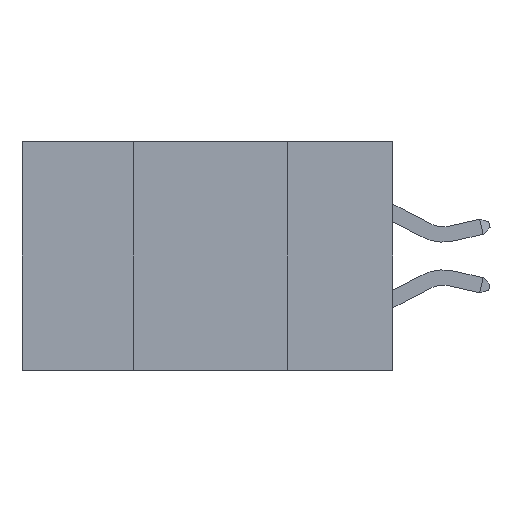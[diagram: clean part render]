
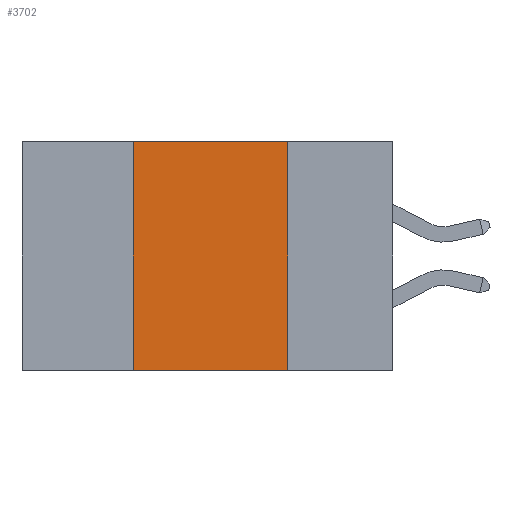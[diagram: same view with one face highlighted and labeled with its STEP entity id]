
A CAD part, left-side view. The second image highlights one B-rep face of the part: STEP entity #3702.
In plain terms, the highlighted planar face has unit normal (-1, 0, 0).
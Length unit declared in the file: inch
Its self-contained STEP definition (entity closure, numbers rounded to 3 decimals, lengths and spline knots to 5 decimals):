
#239 = EDGE_CURVE ( 'NONE', #18527, #651, #13821, .T. ) ;
#514 = DIRECTION ( 'NONE',  ( 0., -1., 0. ) ) ;
#651 = VERTEX_POINT ( 'NONE', #6823 ) ;
#1401 = ORIENTED_EDGE ( 'NONE', *, *, #239, .F. ) ;
#1610 = DIRECTION ( 'NONE',  ( 0., 0., -1. ) ) ;
#1718 = CARTESIAN_POINT ( 'NONE',  ( 0., 0.17, 0. ) ) ;
#1880 = VECTOR ( 'NONE', #3197, 39.37008 ) ;
#1948 = EDGE_CURVE ( 'NONE', #651, #14183, #6397, .T. ) ;
#2410 = VECTOR ( 'NONE', #20404, 39.37008 ) ;
#2916 = CARTESIAN_POINT ( 'NONE',  ( 0., 0.42, 0. ) ) ;
#3197 = DIRECTION ( 'NONE',  ( 0., 0., -1. ) ) ;
#3702 = ADVANCED_FACE ( 'NONE', ( #20665 ), #8839, .F. ) ;
#4089 = VECTOR ( 'NONE', #13491, 39.37008 ) ;
#4586 = VECTOR ( 'NONE', #514, 39.37008 ) ;
#6397 = LINE ( 'NONE', #11805, #2410 ) ;
#6621 = ORIENTED_EDGE ( 'NONE', *, *, #15711, .F. ) ;
#6769 = DIRECTION ( 'NONE',  ( 1., 0., 0. ) ) ;
#6823 = CARTESIAN_POINT ( 'NONE',  ( 0., 0.42, 0. ) ) ;
#7909 = CARTESIAN_POINT ( 'NONE',  ( 0., 0.17, 0. ) ) ;
#8455 = CARTESIAN_POINT ( 'NONE',  ( 0., 0.42, -0.37 ) ) ;
#8602 = AXIS2_PLACEMENT_3D ( 'NONE', #10235, #6769, #1610 ) ;
#8839 = PLANE ( 'NONE',  #8602 ) ;
#10000 = EDGE_CURVE ( 'NONE', #18527, #14753, #19574, .T. ) ;
#10235 = CARTESIAN_POINT ( 'NONE',  ( 0., 0.6, 0. ) ) ;
#10469 = ORIENTED_EDGE ( 'NONE', *, *, #1948, .F. ) ;
#11760 = CARTESIAN_POINT ( 'NONE',  ( 0., 0.17, -0.37 ) ) ;
#11805 = CARTESIAN_POINT ( 'NONE',  ( 0., 0.6, 0. ) ) ;
#13491 = DIRECTION ( 'NONE',  ( 0., 0., 1. ) ) ;
#13821 = LINE ( 'NONE', #2916, #4089 ) ;
#14183 = VERTEX_POINT ( 'NONE', #7909 ) ;
#14753 = VERTEX_POINT ( 'NONE', #11760 ) ;
#15362 = LINE ( 'NONE', #1718, #1880 ) ;
#15711 = EDGE_CURVE ( 'NONE', #14183, #14753, #15362, .T. ) ;
#16231 = CARTESIAN_POINT ( 'NONE',  ( 0., 0.6, -0.37 ) ) ;
#17117 = ORIENTED_EDGE ( 'NONE', *, *, #10000, .T. ) ;
#17172 = EDGE_LOOP ( 'NONE', ( #6621, #10469, #1401, #17117 ) ) ;
#18527 = VERTEX_POINT ( 'NONE', #8455 ) ;
#19574 = LINE ( 'NONE', #16231, #4586 ) ;
#20404 = DIRECTION ( 'NONE',  ( 0., -1., 0. ) ) ;
#20665 = FACE_OUTER_BOUND ( 'NONE', #17172, .T. ) ;
